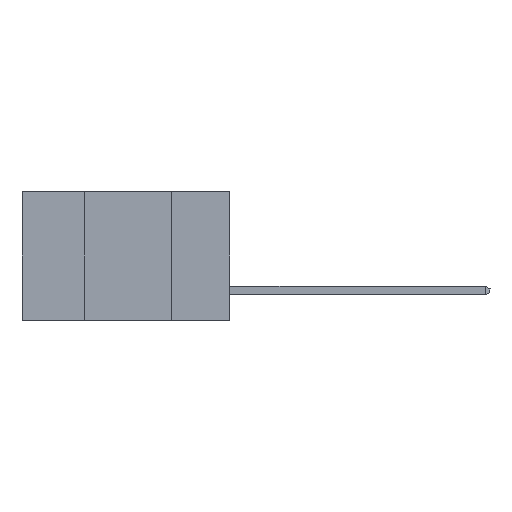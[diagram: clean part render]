
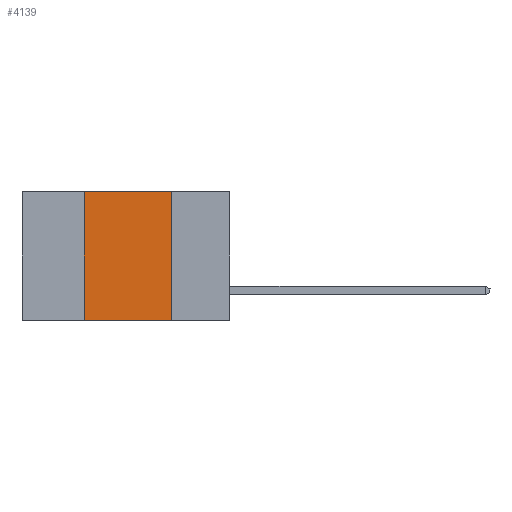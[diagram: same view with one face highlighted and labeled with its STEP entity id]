
A CAD part, left-side view. The second image highlights one B-rep face of the part: STEP entity #4139.
In plain terms, the highlighted planar face has unit normal (-1, 0, 0).
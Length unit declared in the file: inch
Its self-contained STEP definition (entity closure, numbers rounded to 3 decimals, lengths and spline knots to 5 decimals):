
#452 = CARTESIAN_POINT ( 'NONE',  ( 0., 0.6, 0. ) ) ;
#603 = CARTESIAN_POINT ( 'NONE',  ( 0., 0.42, -0.37 ) ) ;
#1134 = EDGE_LOOP ( 'NONE', ( #7836, #7942, #11851, #1656 ) ) ;
#1505 = DIRECTION ( 'NONE',  ( 1., 0., 0. ) ) ;
#1656 = ORIENTED_EDGE ( 'NONE', *, *, #8557, .T. ) ;
#1839 = LINE ( 'NONE', #4188, #9123 ) ;
#2255 = CARTESIAN_POINT ( 'NONE',  ( 0., 0.6, -0.37 ) ) ;
#2824 = VERTEX_POINT ( 'NONE', #3927 ) ;
#3648 = LINE ( 'NONE', #2255, #9060 ) ;
#3927 = CARTESIAN_POINT ( 'NONE',  ( 0., 0.17, 0. ) ) ;
#4139 = ADVANCED_FACE ( 'NONE', ( #12096 ), #9988, .F. ) ;
#4188 = CARTESIAN_POINT ( 'NONE',  ( 0., 0.42, -0.37 ) ) ;
#4427 = CARTESIAN_POINT ( 'NONE',  ( 0., 0.42, 0. ) ) ;
#5068 = VECTOR ( 'NONE', #13484, 39.37008 ) ;
#5692 = VERTEX_POINT ( 'NONE', #4427 ) ;
#6385 = EDGE_CURVE ( 'NONE', #5692, #2824, #13642, .T. ) ;
#6430 = LINE ( 'NONE', #11295, #8440 ) ;
#7751 = CARTESIAN_POINT ( 'NONE',  ( 0., 0.17, -0.37 ) ) ;
#7836 = ORIENTED_EDGE ( 'NONE', *, *, #15181, .F. ) ;
#7942 = ORIENTED_EDGE ( 'NONE', *, *, #6385, .F. ) ;
#8440 = VECTOR ( 'NONE', #9977, 39.37008 ) ;
#8557 = EDGE_CURVE ( 'NONE', #10525, #10268, #3648, .T. ) ;
#8574 = CARTESIAN_POINT ( 'NONE',  ( 0., 0.6, 0. ) ) ;
#8985 = DIRECTION ( 'NONE',  ( 0., 0., 1. ) ) ;
#9060 = VECTOR ( 'NONE', #9706, 39.37008 ) ;
#9123 = VECTOR ( 'NONE', #8985, 39.37008 ) ;
#9327 = AXIS2_PLACEMENT_3D ( 'NONE', #8574, #1505, #10848 ) ;
#9706 = DIRECTION ( 'NONE',  ( 0., -1., 0. ) ) ;
#9977 = DIRECTION ( 'NONE',  ( 0., 0., -1. ) ) ;
#9988 = PLANE ( 'NONE',  #9327 ) ;
#10215 = EDGE_CURVE ( 'NONE', #10525, #5692, #1839, .T. ) ;
#10268 = VERTEX_POINT ( 'NONE', #7751 ) ;
#10525 = VERTEX_POINT ( 'NONE', #603 ) ;
#10848 = DIRECTION ( 'NONE',  ( 0., 0., -1. ) ) ;
#11295 = CARTESIAN_POINT ( 'NONE',  ( 0., 0.17, -0.37 ) ) ;
#11851 = ORIENTED_EDGE ( 'NONE', *, *, #10215, .F. ) ;
#12096 = FACE_OUTER_BOUND ( 'NONE', #1134, .T. ) ;
#13484 = DIRECTION ( 'NONE',  ( 0., -1., 0. ) ) ;
#13642 = LINE ( 'NONE', #452, #5068 ) ;
#15181 = EDGE_CURVE ( 'NONE', #2824, #10268, #6430, .T. ) ;
